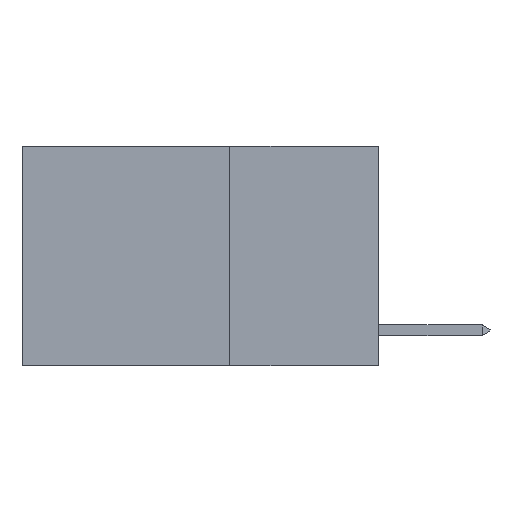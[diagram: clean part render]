
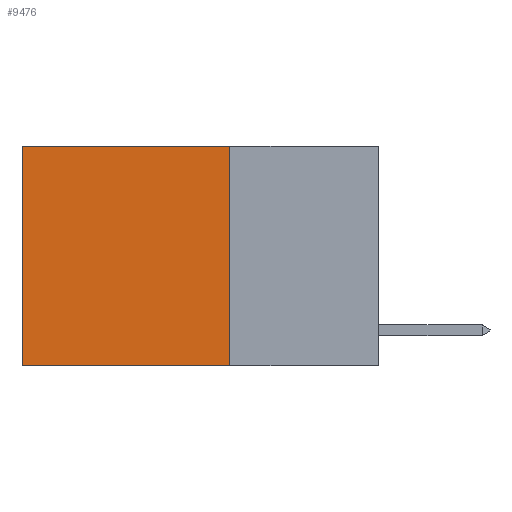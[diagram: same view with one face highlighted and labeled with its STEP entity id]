
A CAD part, left-side view. The second image highlights one B-rep face of the part: STEP entity #9476.
In plain terms, the highlighted planar face has unit normal (-1, 0, 0).
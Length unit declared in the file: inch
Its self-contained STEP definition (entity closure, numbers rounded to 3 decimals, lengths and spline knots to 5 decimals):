
#1518 = ORIENTED_EDGE ( 'NONE', *, *, #17681, .T. ) ;
#1703 = VECTOR ( 'NONE', #19941, 39.37008 ) ;
#2991 = VECTOR ( 'NONE', #15877, 39.37008 ) ;
#3264 = VECTOR ( 'NONE', #18623, 39.37008 ) ;
#3597 = VERTEX_POINT ( 'NONE', #18309 ) ;
#4078 = EDGE_CURVE ( 'NONE', #21694, #9513, #15487, .T. ) ;
#4337 = VERTEX_POINT ( 'NONE', #6506 ) ;
#6155 = ORIENTED_EDGE ( 'NONE', *, *, #4078, .F. ) ;
#6506 = CARTESIAN_POINT ( 'NONE',  ( 0.2625, 0.6, -0.37 ) ) ;
#7988 = EDGE_LOOP ( 'NONE', ( #20851, #20153, #6155, #1518 ) ) ;
#8379 = CARTESIAN_POINT ( 'NONE',  ( 0.2625, 0.25, 0. ) ) ;
#9332 = CARTESIAN_POINT ( 'NONE',  ( 0.2625, 0.25, 0. ) ) ;
#9476 = ADVANCED_FACE ( 'NONE', ( #17983 ), #18702, .F. ) ;
#9513 = VERTEX_POINT ( 'NONE', #22168 ) ;
#10125 = DIRECTION ( 'NONE',  ( 0., 0., -1. ) ) ;
#10947 = LINE ( 'NONE', #16540, #1703 ) ;
#11305 = EDGE_CURVE ( 'NONE', #9513, #4337, #17117, .T. ) ;
#11541 = EDGE_CURVE ( 'NONE', #3597, #4337, #16831, .T. ) ;
#11804 = CARTESIAN_POINT ( 'NONE',  ( 0.2625, 0.25, -0.37 ) ) ;
#12390 = CARTESIAN_POINT ( 'NONE',  ( 0.2625, 0.6, 0. ) ) ;
#15487 = LINE ( 'NONE', #9332, #19481 ) ;
#15877 = DIRECTION ( 'NONE',  ( 0., 0., -1. ) ) ;
#16540 = CARTESIAN_POINT ( 'NONE',  ( 0.2625, 0.25, 0. ) ) ;
#16831 = LINE ( 'NONE', #12390, #2991 ) ;
#17117 = LINE ( 'NONE', #11804, #3264 ) ;
#17681 = EDGE_CURVE ( 'NONE', #21694, #3597, #10947, .T. ) ;
#17914 = DIRECTION ( 'NONE',  ( 0., 0., -1. ) ) ;
#17967 = CARTESIAN_POINT ( 'NONE',  ( 0.2625, 0.25, 0. ) ) ;
#17983 = FACE_OUTER_BOUND ( 'NONE', #7988, .T. ) ;
#18087 = AXIS2_PLACEMENT_3D ( 'NONE', #8379, #20400, #10125 ) ;
#18309 = CARTESIAN_POINT ( 'NONE',  ( 0.2625, 0.6, 0. ) ) ;
#18623 = DIRECTION ( 'NONE',  ( 0., 1., 0. ) ) ;
#18702 = PLANE ( 'NONE',  #18087 ) ;
#19481 = VECTOR ( 'NONE', #17914, 39.37008 ) ;
#19941 = DIRECTION ( 'NONE',  ( 0., 1., 0. ) ) ;
#20153 = ORIENTED_EDGE ( 'NONE', *, *, #11305, .F. ) ;
#20400 = DIRECTION ( 'NONE',  ( 1., 0., 0. ) ) ;
#20851 = ORIENTED_EDGE ( 'NONE', *, *, #11541, .T. ) ;
#21694 = VERTEX_POINT ( 'NONE', #17967 ) ;
#22168 = CARTESIAN_POINT ( 'NONE',  ( 0.2625, 0.25, -0.37 ) ) ;
